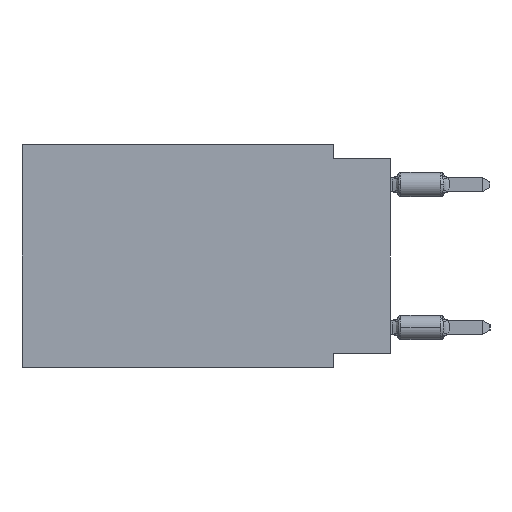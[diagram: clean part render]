
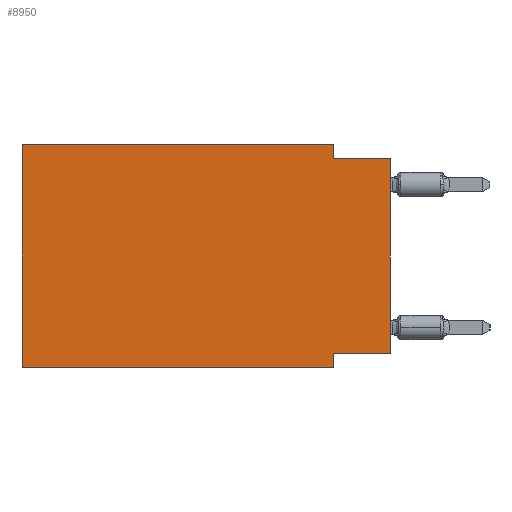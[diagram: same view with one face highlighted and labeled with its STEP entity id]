
A CAD part, left-side view. The second image highlights one B-rep face of the part: STEP entity #8950.
In plain terms, the highlighted planar face has unit normal (-1, 0, 0).
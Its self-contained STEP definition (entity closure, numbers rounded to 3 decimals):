
#66 = DIRECTION ( 'NONE',  ( 0., -1., 0. ) ) ;
#287 = ORIENTED_EDGE ( 'NONE', *, *, #27515, .F. ) ;
#587 = LINE ( 'NONE', #14161, #42132 ) ;
#643 = CARTESIAN_POINT ( 'NONE',  ( 0., 16.383, 0. ) ) ;
#2412 = VECTOR ( 'NONE', #39862, 1000. ) ;
#3226 = EDGE_CURVE ( 'NONE', #35905, #30217, #7085, .T. ) ;
#3448 = CARTESIAN_POINT ( 'NONE',  ( 0., 2.54, 0. ) ) ;
#3580 = VECTOR ( 'NONE', #29312, 1000. ) ;
#3848 = VERTEX_POINT ( 'NONE', #27184 ) ;
#3976 = DIRECTION ( 'NONE',  ( 0., 0., -1. ) ) ;
#4759 = VERTEX_POINT ( 'NONE', #9734 ) ;
#4927 = LINE ( 'NONE', #12034, #10915 ) ;
#6897 = VERTEX_POINT ( 'NONE', #11359 ) ;
#7085 = LINE ( 'NONE', #643, #29409 ) ;
#7184 = VERTEX_POINT ( 'NONE', #20436 ) ;
#7663 = CARTESIAN_POINT ( 'NONE',  ( 0., 0., 0. ) ) ;
#8950 = ADVANCED_FACE ( 'NONE', ( #10385 ), #24388, .F. ) ;
#9734 = CARTESIAN_POINT ( 'NONE',  ( 0., 0., -9.271 ) ) ;
#10385 = FACE_OUTER_BOUND ( 'NONE', #26475, .T. ) ;
#10464 = EDGE_CURVE ( 'NONE', #4759, #15007, #38686, .T. ) ;
#10915 = VECTOR ( 'NONE', #31852, 1000. ) ;
#11359 = CARTESIAN_POINT ( 'NONE',  ( 0., 2.54, -9.906 ) ) ;
#11454 = VERTEX_POINT ( 'NONE', #25734 ) ;
#12034 = CARTESIAN_POINT ( 'NONE',  ( 0., 2.54, 0. ) ) ;
#12523 = EDGE_CURVE ( 'NONE', #15007, #6897, #31782, .T. ) ;
#13975 = CARTESIAN_POINT ( 'NONE',  ( 0., 2.54, -9.271 ) ) ;
#14161 = CARTESIAN_POINT ( 'NONE',  ( 0., 16.383, 0. ) ) ;
#14867 = CARTESIAN_POINT ( 'NONE',  ( 0., 2.54, -9.906 ) ) ;
#15007 = VERTEX_POINT ( 'NONE', #13975 ) ;
#17710 = DIRECTION ( 'NONE',  ( 0., 0., -1. ) ) ;
#18419 = ORIENTED_EDGE ( 'NONE', *, *, #12523, .F. ) ;
#18811 = EDGE_CURVE ( 'NONE', #30217, #11454, #4927, .T. ) ;
#20436 = CARTESIAN_POINT ( 'NONE',  ( 0., 16.383, -9.906 ) ) ;
#20537 = LINE ( 'NONE', #40120, #34109 ) ;
#21053 = DIRECTION ( 'NONE',  ( 1., 0., 0. ) ) ;
#21870 = ORIENTED_EDGE ( 'NONE', *, *, #31079, .T. ) ;
#23167 = VECTOR ( 'NONE', #3976, 1000. ) ;
#23565 = ORIENTED_EDGE ( 'NONE', *, *, #42282, .F. ) ;
#24388 = PLANE ( 'NONE',  #36550 ) ;
#25734 = CARTESIAN_POINT ( 'NONE',  ( 0., 2.54, -0.635 ) ) ;
#26306 = LINE ( 'NONE', #35904, #2412 ) ;
#26475 = EDGE_LOOP ( 'NONE', ( #35171, #23565, #28752, #38382, #287, #21870, #18419, #39018 ) ) ;
#27184 = CARTESIAN_POINT ( 'NONE',  ( 0., 0., -0.635 ) ) ;
#27515 = EDGE_CURVE ( 'NONE', #7184, #35905, #587, .T. ) ;
#27725 = DIRECTION ( 'NONE',  ( 0., 0., 1. ) ) ;
#28708 = VECTOR ( 'NONE', #30379, 1000. ) ;
#28752 = ORIENTED_EDGE ( 'NONE', *, *, #18811, .F. ) ;
#29312 = DIRECTION ( 'NONE',  ( 0., 1., 0. ) ) ;
#29409 = VECTOR ( 'NONE', #31348, 1000. ) ;
#30217 = VERTEX_POINT ( 'NONE', #3448 ) ;
#30379 = DIRECTION ( 'NONE',  ( 0., 0., 1. ) ) ;
#30821 = EDGE_CURVE ( 'NONE', #4759, #3848, #37921, .T. ) ;
#31079 = EDGE_CURVE ( 'NONE', #7184, #6897, #26306, .T. ) ;
#31348 = DIRECTION ( 'NONE',  ( 0., -1., 0. ) ) ;
#31782 = LINE ( 'NONE', #14867, #23167 ) ;
#31852 = DIRECTION ( 'NONE',  ( 0., 0., -1. ) ) ;
#34109 = VECTOR ( 'NONE', #66, 1000. ) ;
#35171 = ORIENTED_EDGE ( 'NONE', *, *, #30821, .T. ) ;
#35904 = CARTESIAN_POINT ( 'NONE',  ( 0., 16.383, -9.906 ) ) ;
#35905 = VERTEX_POINT ( 'NONE', #40577 ) ;
#36004 = CARTESIAN_POINT ( 'NONE',  ( 0., 0., -9.271 ) ) ;
#36550 = AXIS2_PLACEMENT_3D ( 'NONE', #37960, #21053, #17710 ) ;
#37921 = LINE ( 'NONE', #7663, #28708 ) ;
#37960 = CARTESIAN_POINT ( 'NONE',  ( 0., 16.383, 0. ) ) ;
#38382 = ORIENTED_EDGE ( 'NONE', *, *, #3226, .F. ) ;
#38686 = LINE ( 'NONE', #36004, #3580 ) ;
#39018 = ORIENTED_EDGE ( 'NONE', *, *, #10464, .F. ) ;
#39862 = DIRECTION ( 'NONE',  ( 0., -1., 0. ) ) ;
#40120 = CARTESIAN_POINT ( 'NONE',  ( 0., 0., -0.635 ) ) ;
#40577 = CARTESIAN_POINT ( 'NONE',  ( 0., 16.383, 0. ) ) ;
#42132 = VECTOR ( 'NONE', #27725, 1000. ) ;
#42282 = EDGE_CURVE ( 'NONE', #11454, #3848, #20537, .T. ) ;
